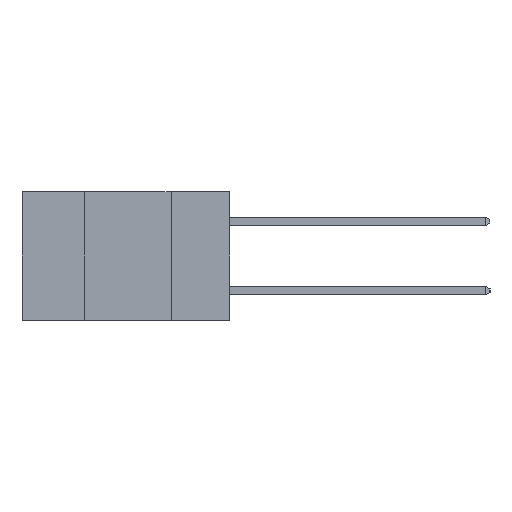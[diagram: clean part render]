
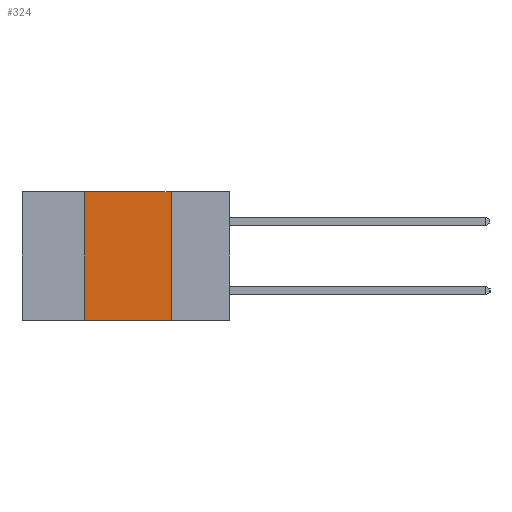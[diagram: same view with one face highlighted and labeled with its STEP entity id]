
A CAD part, left-side view. The second image highlights one B-rep face of the part: STEP entity #324.
In plain terms, the highlighted planar face has unit normal (-1, 0, 0).
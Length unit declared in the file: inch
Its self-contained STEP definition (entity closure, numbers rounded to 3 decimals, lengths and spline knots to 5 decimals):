
#324 = ADVANCED_FACE ( 'NONE', ( #1095 ), #4411, .F. ) ;
#607 = VECTOR ( 'NONE', #8778, 39.37008 ) ;
#917 = CARTESIAN_POINT ( 'NONE',  ( 0., 0.6, -0.37 ) ) ;
#932 = EDGE_CURVE ( 'NONE', #8272, #11364, #7883, .T. ) ;
#1095 = FACE_OUTER_BOUND ( 'NONE', #2005, .T. ) ;
#1818 = EDGE_CURVE ( 'NONE', #8272, #5294, #7861, .T. ) ;
#2005 = EDGE_LOOP ( 'NONE', ( #2908, #10180, #5071, #11223 ) ) ;
#2859 = LINE ( 'NONE', #5923, #607 ) ;
#2908 = ORIENTED_EDGE ( 'NONE', *, *, #7402, .F. ) ;
#2993 = DIRECTION ( 'NONE',  ( 1., 0., 0. ) ) ;
#3433 = CARTESIAN_POINT ( 'NONE',  ( 0., 0.17, 0. ) ) ;
#3850 = CARTESIAN_POINT ( 'NONE',  ( 0., 0.6, 0. ) ) ;
#4411 = PLANE ( 'NONE',  #7539 ) ;
#4486 = VERTEX_POINT ( 'NONE', #3433 ) ;
#4792 = EDGE_CURVE ( 'NONE', #11364, #4486, #10035, .T. ) ;
#4913 = VECTOR ( 'NONE', #9654, 39.37008 ) ;
#5071 = ORIENTED_EDGE ( 'NONE', *, *, #932, .F. ) ;
#5282 = VECTOR ( 'NONE', #7677, 39.37008 ) ;
#5294 = VERTEX_POINT ( 'NONE', #12375 ) ;
#5306 = VECTOR ( 'NONE', #9275, 39.37008 ) ;
#5923 = CARTESIAN_POINT ( 'NONE',  ( 0., 0.17, -0.37 ) ) ;
#7402 = EDGE_CURVE ( 'NONE', #4486, #5294, #2859, .T. ) ;
#7539 = AXIS2_PLACEMENT_3D ( 'NONE', #12076, #2993, #8270 ) ;
#7677 = DIRECTION ( 'NONE',  ( 0., -1., 0. ) ) ;
#7861 = LINE ( 'NONE', #917, #5282 ) ;
#7883 = LINE ( 'NONE', #10598, #5306 ) ;
#8270 = DIRECTION ( 'NONE',  ( 0., 0., -1. ) ) ;
#8272 = VERTEX_POINT ( 'NONE', #11128 ) ;
#8778 = DIRECTION ( 'NONE',  ( 0., 0., -1. ) ) ;
#9275 = DIRECTION ( 'NONE',  ( 0., 0., 1. ) ) ;
#9654 = DIRECTION ( 'NONE',  ( 0., -1., 0. ) ) ;
#10035 = LINE ( 'NONE', #3850, #4913 ) ;
#10180 = ORIENTED_EDGE ( 'NONE', *, *, #4792, .F. ) ;
#10598 = CARTESIAN_POINT ( 'NONE',  ( 0., 0.42, -0.37 ) ) ;
#11128 = CARTESIAN_POINT ( 'NONE',  ( 0., 0.42, -0.37 ) ) ;
#11223 = ORIENTED_EDGE ( 'NONE', *, *, #1818, .T. ) ;
#11364 = VERTEX_POINT ( 'NONE', #11409 ) ;
#11409 = CARTESIAN_POINT ( 'NONE',  ( 0., 0.42, 0. ) ) ;
#12076 = CARTESIAN_POINT ( 'NONE',  ( 0., 0.6, 0. ) ) ;
#12375 = CARTESIAN_POINT ( 'NONE',  ( 0., 0.17, -0.37 ) ) ;
